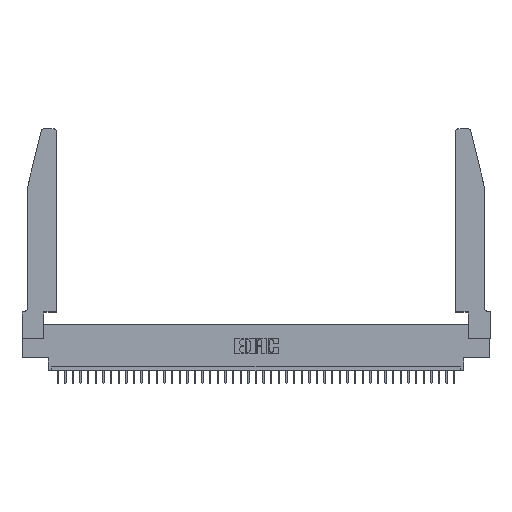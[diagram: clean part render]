
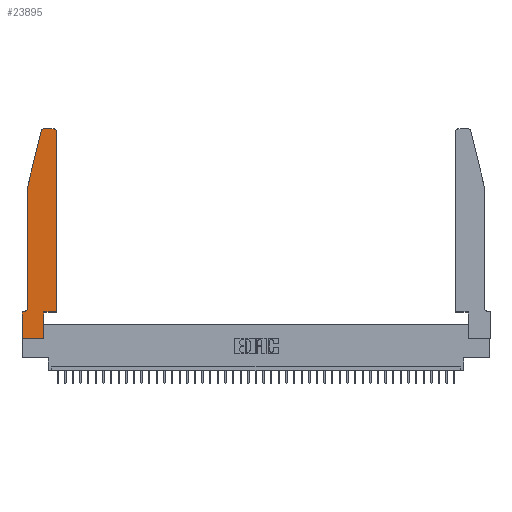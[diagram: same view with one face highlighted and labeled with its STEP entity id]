
A CAD part, top view. The second image highlights one B-rep face of the part: STEP entity #23895.
In plain terms, the highlighted planar face has unit normal (0, 0, 1).
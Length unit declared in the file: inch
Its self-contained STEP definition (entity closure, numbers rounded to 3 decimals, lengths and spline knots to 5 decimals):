
#1319 = DIRECTION ( 'NONE',  ( -1., 0., 0. ) ) ;
#1681 = VECTOR ( 'NONE', #37500, 39.37008 ) ;
#2772 = CARTESIAN_POINT ( 'NONE',  ( 0., 0.35, 0.37 ) ) ;
#2944 = EDGE_LOOP ( 'NONE', ( #30627, #24148, #25434, #30296, #34247, #33596, #21937, #10665, #9363, #21616, #9790, #4041 ) ) ;
#4041 = ORIENTED_EDGE ( 'NONE', *, *, #42750, .T. ) ;
#4865 = CARTESIAN_POINT ( 'NONE',  ( 0., 0., 0.37 ) ) ;
#5026 = LINE ( 'NONE', #14855, #34251 ) ;
#6086 = CARTESIAN_POINT ( 'NONE',  ( 0.2865, 0.35, 0.37 ) ) ;
#6501 = CARTESIAN_POINT ( 'NONE',  ( 0., 0.35, 0.37 ) ) ;
#6549 = DIRECTION ( 'NONE',  ( -1., 0., 0. ) ) ;
#6603 = EDGE_CURVE ( 'NONE', #35299, #10146, #38127, .T. ) ;
#6704 = VERTEX_POINT ( 'NONE', #22925 ) ;
#6969 = EDGE_CURVE ( 'NONE', #19697, #25848, #41770, .T. ) ;
#7666 = CARTESIAN_POINT ( 'NONE',  ( 0., 0., 0.37 ) ) ;
#8213 = CARTESIAN_POINT ( 'NONE',  ( 0.0055, 0.42, 0.37 ) ) ;
#8723 = AXIS2_PLACEMENT_3D ( 'NONE', #8213, #21451, #38167 ) ;
#9363 = ORIENTED_EDGE ( 'NONE', *, *, #38719, .T. ) ;
#9402 = VERTEX_POINT ( 'NONE', #39031 ) ;
#9790 = ORIENTED_EDGE ( 'NONE', *, *, #6603, .T. ) ;
#9884 = LINE ( 'NONE', #36048, #38084 ) ;
#10146 = VERTEX_POINT ( 'NONE', #22769 ) ;
#10172 = EDGE_CURVE ( 'NONE', #42918, #35299, #19583, .T. ) ;
#10294 = CARTESIAN_POINT ( 'NONE',  ( 0.25487, 2.72718, 0.37 ) ) ;
#10665 = ORIENTED_EDGE ( 'NONE', *, *, #19551, .T. ) ;
#11485 = CARTESIAN_POINT ( 'NONE',  ( 0.284, 2.72, 0.37 ) ) ;
#12178 = VECTOR ( 'NONE', #13414, 39.37008 ) ;
#12438 = CIRCLE ( 'NONE', #8723, 0.07 ) ;
#13324 = VECTOR ( 'NONE', #39348, 39.37008 ) ;
#13414 = DIRECTION ( 'NONE',  ( -0.239, -0.971, 0. ) ) ;
#14167 = VERTEX_POINT ( 'NONE', #36398 ) ;
#14536 = EDGE_CURVE ( 'NONE', #9402, #19697, #5026, .T. ) ;
#14537 = CARTESIAN_POINT ( 'NONE',  ( 0.2865, 0.35, 0.37 ) ) ;
#14855 = CARTESIAN_POINT ( 'NONE',  ( 0.2605, 2.75, 0.37 ) ) ;
#15350 = LINE ( 'NONE', #7666, #1681 ) ;
#15870 = VERTEX_POINT ( 'NONE', #38011 ) ;
#16526 = EDGE_CURVE ( 'NONE', #23395, #30256, #33367, .T. ) ;
#17592 = DIRECTION ( 'NONE',  ( 1., 0., 0. ) ) ;
#17676 = VECTOR ( 'NONE', #6549, 39.37008 ) ;
#17941 = CARTESIAN_POINT ( 'NONE',  ( 0.284, 2.75, 0.37 ) ) ;
#18231 = DIRECTION ( 'NONE',  ( 0., 0., 1. ) ) ;
#18685 = CARTESIAN_POINT ( 'NONE',  ( 0.0055, 0.35, 0.37 ) ) ;
#18992 = DIRECTION ( 'NONE',  ( 0., -1., 0. ) ) ;
#19308 = LINE ( 'NONE', #14537, #35465 ) ;
#19551 = EDGE_CURVE ( 'NONE', #26411, #15870, #15350, .T. ) ;
#19583 = LINE ( 'NONE', #39785, #13324 ) ;
#19697 = VERTEX_POINT ( 'NONE', #17941 ) ;
#21451 = DIRECTION ( 'NONE',  ( 0., 0., -1. ) ) ;
#21616 = ORIENTED_EDGE ( 'NONE', *, *, #10172, .T. ) ;
#21937 = ORIENTED_EDGE ( 'NONE', *, *, #33286, .T. ) ;
#22538 = DIRECTION ( 'NONE',  ( 0., 1., 0. ) ) ;
#22769 = CARTESIAN_POINT ( 'NONE',  ( 0.4505, 2.72, 0.37 ) ) ;
#22856 = CARTESIAN_POINT ( 'NONE',  ( 0.0755, 0.35, 0.37 ) ) ;
#22925 = CARTESIAN_POINT ( 'NONE',  ( 0.0755, 0.42, 0.37 ) ) ;
#23395 = VERTEX_POINT ( 'NONE', #18685 ) ;
#23745 = EDGE_CURVE ( 'NONE', #14167, #6704, #9884, .T. ) ;
#23895 = ADVANCED_FACE ( 'NONE', ( #25081 ), #24904, .T. ) ;
#24148 = ORIENTED_EDGE ( 'NONE', *, *, #6969, .T. ) ;
#24377 = AXIS2_PLACEMENT_3D ( 'NONE', #41453, #18231, #41597 ) ;
#24904 = PLANE ( 'NONE',  #31348 ) ;
#24934 = EDGE_CURVE ( 'NONE', #6704, #23395, #12438, .T. ) ;
#25081 = FACE_OUTER_BOUND ( 'NONE', #2944, .T. ) ;
#25125 = CARTESIAN_POINT ( 'NONE',  ( 0., 0., 0.37 ) ) ;
#25434 = ORIENTED_EDGE ( 'NONE', *, *, #36811, .T. ) ;
#25848 = VERTEX_POINT ( 'NONE', #10294 ) ;
#26411 = VERTEX_POINT ( 'NONE', #4865 ) ;
#28644 = LINE ( 'NONE', #25125, #32843 ) ;
#30256 = VERTEX_POINT ( 'NONE', #6501 ) ;
#30296 = ORIENTED_EDGE ( 'NONE', *, *, #23745, .T. ) ;
#30627 = ORIENTED_EDGE ( 'NONE', *, *, #14536, .T. ) ;
#31348 = AXIS2_PLACEMENT_3D ( 'NONE', #2772, #36688, #40201 ) ;
#32083 = DIRECTION ( 'NONE',  ( 0., -1., 0. ) ) ;
#32843 = VECTOR ( 'NONE', #32083, 39.37008 ) ;
#33286 = EDGE_CURVE ( 'NONE', #30256, #26411, #28644, .T. ) ;
#33367 = LINE ( 'NONE', #22856, #17676 ) ;
#33386 = CARTESIAN_POINT ( 'NONE',  ( 0.0755, 2., 0.37 ) ) ;
#33596 = ORIENTED_EDGE ( 'NONE', *, *, #16526, .T. ) ;
#33997 = CIRCLE ( 'NONE', #24377, 0.03 ) ;
#34247 = ORIENTED_EDGE ( 'NONE', *, *, #24934, .T. ) ;
#34251 = VECTOR ( 'NONE', #1319, 39.37008 ) ;
#34650 = DIRECTION ( 'NONE',  ( 0., 0., 1. ) ) ;
#34802 = DIRECTION ( 'NONE',  ( 0., 1., 0. ) ) ;
#35096 = CARTESIAN_POINT ( 'NONE',  ( 0.4505, 0.35, 0.37 ) ) ;
#35299 = VERTEX_POINT ( 'NONE', #35096 ) ;
#35465 = VECTOR ( 'NONE', #34802, 39.37008 ) ;
#36048 = CARTESIAN_POINT ( 'NONE',  ( 0.0755, 2., 0.37 ) ) ;
#36398 = CARTESIAN_POINT ( 'NONE',  ( 0.0755, 2., 0.37 ) ) ;
#36688 = DIRECTION ( 'NONE',  ( 0., 0., 1. ) ) ;
#36811 = EDGE_CURVE ( 'NONE', #25848, #14167, #40854, .T. ) ;
#37500 = DIRECTION ( 'NONE',  ( 1., 0., 0. ) ) ;
#38011 = CARTESIAN_POINT ( 'NONE',  ( 0.2865, 0., 0.37 ) ) ;
#38084 = VECTOR ( 'NONE', #18992, 39.37008 ) ;
#38127 = LINE ( 'NONE', #42483, #38665 ) ;
#38167 = DIRECTION ( 'NONE',  ( -1., 0., 0. ) ) ;
#38665 = VECTOR ( 'NONE', #22538, 39.37008 ) ;
#38719 = EDGE_CURVE ( 'NONE', #15870, #42918, #19308, .T. ) ;
#39031 = CARTESIAN_POINT ( 'NONE',  ( 0.4205, 2.75, 0.37 ) ) ;
#39348 = DIRECTION ( 'NONE',  ( 1., 0., 0. ) ) ;
#39785 = CARTESIAN_POINT ( 'NONE',  ( 0.4505, 0.35, 0.37 ) ) ;
#40201 = DIRECTION ( 'NONE',  ( 1., 0., 0. ) ) ;
#40854 = LINE ( 'NONE', #33386, #12178 ) ;
#41341 = AXIS2_PLACEMENT_3D ( 'NONE', #11485, #34650, #17592 ) ;
#41453 = CARTESIAN_POINT ( 'NONE',  ( 0.4205, 2.72, 0.37 ) ) ;
#41597 = DIRECTION ( 'NONE',  ( 1., 0., 0. ) ) ;
#41770 = CIRCLE ( 'NONE', #41341, 0.03 ) ;
#42483 = CARTESIAN_POINT ( 'NONE',  ( 0.4505, 0.35, 0.37 ) ) ;
#42750 = EDGE_CURVE ( 'NONE', #10146, #9402, #33997, .T. ) ;
#42918 = VERTEX_POINT ( 'NONE', #6086 ) ;
